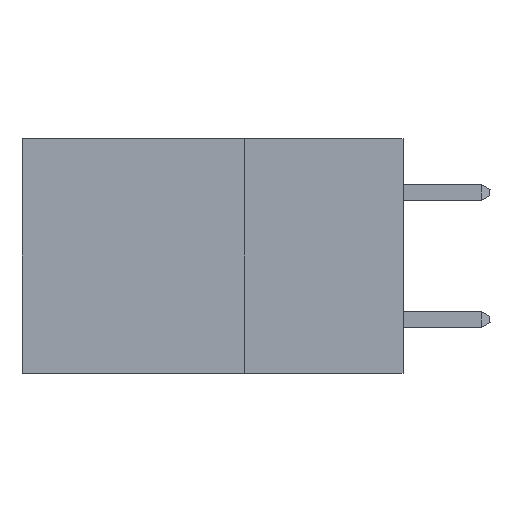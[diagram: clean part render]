
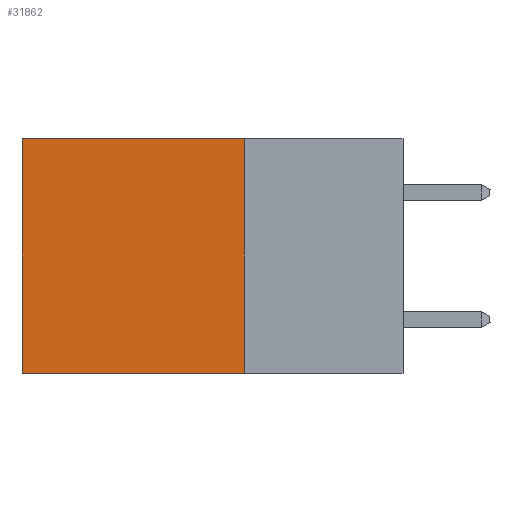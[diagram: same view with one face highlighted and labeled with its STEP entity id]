
A CAD part, left-side view. The second image highlights one B-rep face of the part: STEP entity #31862.
In plain terms, the highlighted planar face has unit normal (-1, 0, 0).
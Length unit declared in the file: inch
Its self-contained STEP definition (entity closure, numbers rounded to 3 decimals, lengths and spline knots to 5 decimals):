
#2842 = VERTEX_POINT ( 'NONE', #22643 ) ;
#3259 = FACE_OUTER_BOUND ( 'NONE', #30387, .T. ) ;
#6552 = EDGE_CURVE ( 'NONE', #26732, #2842, #26984, .T. ) ;
#6745 = DIRECTION ( 'NONE',  ( 0., 0., -1. ) ) ;
#7019 = DIRECTION ( 'NONE',  ( 0., 1., 0. ) ) ;
#7277 = CARTESIAN_POINT ( 'NONE',  ( 0.2875, 0.25, 0. ) ) ;
#10285 = CARTESIAN_POINT ( 'NONE',  ( 0.2875, 0.25, 0. ) ) ;
#10995 = VECTOR ( 'NONE', #32610, 39.37008 ) ;
#12526 = VECTOR ( 'NONE', #7019, 39.37008 ) ;
#13846 = CARTESIAN_POINT ( 'NONE',  ( 0.2875, 0.25, 0. ) ) ;
#14521 = ORIENTED_EDGE ( 'NONE', *, *, #43089, .F. ) ;
#15487 = ORIENTED_EDGE ( 'NONE', *, *, #27893, .T. ) ;
#16055 = LINE ( 'NONE', #18007, #12526 ) ;
#18007 = CARTESIAN_POINT ( 'NONE',  ( 0.2875, 0.25, 0. ) ) ;
#19422 = CARTESIAN_POINT ( 'NONE',  ( 0.2875, 0.6, -0.37 ) ) ;
#19785 = AXIS2_PLACEMENT_3D ( 'NONE', #10285, #43985, #6745 ) ;
#20828 = LINE ( 'NONE', #39938, #10995 ) ;
#21177 = VECTOR ( 'NONE', #43652, 39.37008 ) ;
#22643 = CARTESIAN_POINT ( 'NONE',  ( 0.2875, 0.25, -0.37 ) ) ;
#26732 = VERTEX_POINT ( 'NONE', #7277 ) ;
#26984 = LINE ( 'NONE', #13846, #21177 ) ;
#27893 = EDGE_CURVE ( 'NONE', #41437, #29331, #44709, .T. ) ;
#28761 = PLANE ( 'NONE',  #19785 ) ;
#29331 = VERTEX_POINT ( 'NONE', #19422 ) ;
#29738 = ORIENTED_EDGE ( 'NONE', *, *, #6552, .F. ) ;
#30387 = EDGE_LOOP ( 'NONE', ( #15487, #14521, #29738, #45536 ) ) ;
#31323 = EDGE_CURVE ( 'NONE', #26732, #41437, #16055, .T. ) ;
#31862 = ADVANCED_FACE ( 'NONE', ( #3259 ), #28761, .F. ) ;
#32610 = DIRECTION ( 'NONE',  ( 0., 1., 0. ) ) ;
#33919 = CARTESIAN_POINT ( 'NONE',  ( 0.2875, 0.6, 0. ) ) ;
#34792 = VECTOR ( 'NONE', #37828, 39.37008 ) ;
#37828 = DIRECTION ( 'NONE',  ( 0., 0., -1. ) ) ;
#39938 = CARTESIAN_POINT ( 'NONE',  ( 0.2875, 0.25, -0.37 ) ) ;
#41437 = VERTEX_POINT ( 'NONE', #44550 ) ;
#43089 = EDGE_CURVE ( 'NONE', #2842, #29331, #20828, .T. ) ;
#43652 = DIRECTION ( 'NONE',  ( 0., 0., -1. ) ) ;
#43985 = DIRECTION ( 'NONE',  ( 1., 0., 0. ) ) ;
#44550 = CARTESIAN_POINT ( 'NONE',  ( 0.2875, 0.6, 0. ) ) ;
#44709 = LINE ( 'NONE', #33919, #34792 ) ;
#45536 = ORIENTED_EDGE ( 'NONE', *, *, #31323, .T. ) ;
